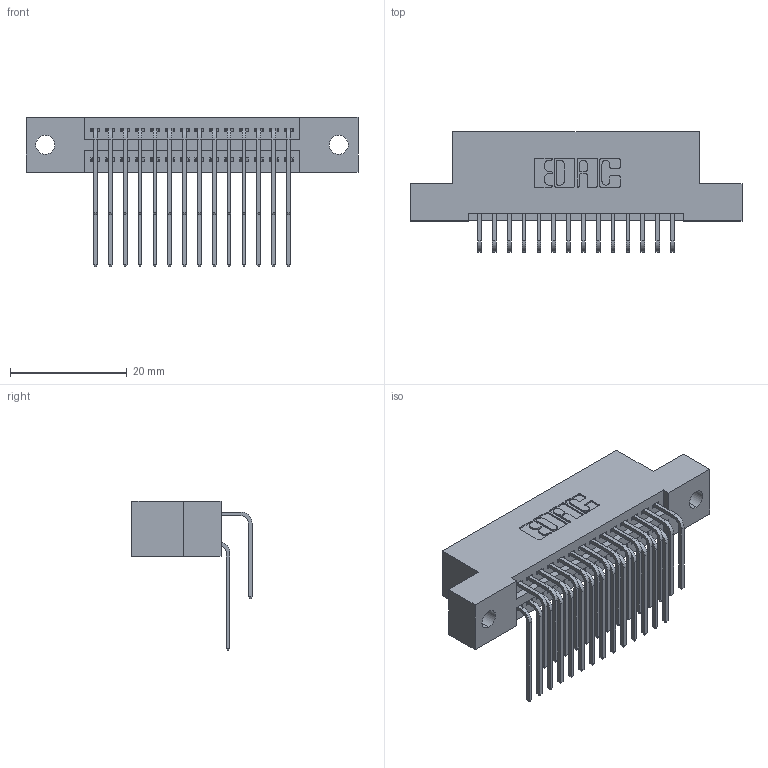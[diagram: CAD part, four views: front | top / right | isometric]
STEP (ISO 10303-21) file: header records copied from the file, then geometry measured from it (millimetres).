
FILE_DESCRIPTION (( 'STEP AP203' ), '1' );
FILE_NAME ('345-028-559-202.STEP', '2018-08-22T23:48:55', ( '' ), ( '' ), 'SwSTEP 2.0', 'SolidWorks 2016', '' );
FILE_SCHEMA (( 'CONFIG_CONTROL_DESIGN' ));
Length unit declared in the file: inch
Products named in the file (4): 345-292-001_558 559 Tail - 1; 345-292-001_559 Tail - 2; 345-028-559-202; 345 Part_Flush Mounting Lugs - 0.128 Dia
Assembly tree (29 placements, depth 2):
  345-028-559-202
    345 Part_Flush Mounting Lugs - 0.128 Dia
    345-292-001_558 559 Tail - 1  x14
    345-292-001_559 Tail - 2  x14
Bounding box: 56.77 x 20.56 x 25.53 mm (x, y, z)
Volume: 5379.5 mm3; surface area: 7896.4 mm2
Topology: 29 solids, 29 shells, 1582 faces, 4681 edges, 3082 vertices
Faces by surface type: plane 1060, cylinder 522
Entity records: 16409 total; most frequent: CARTESIAN_POINT 2823, ORIENTED_EDGE 2706, DIRECTION 2497, EDGE_CURVE 1353, LINE 1125, VECTOR 1125, VERTEX_POINT 898, AXIS2_PLACEMENT_3D 686
